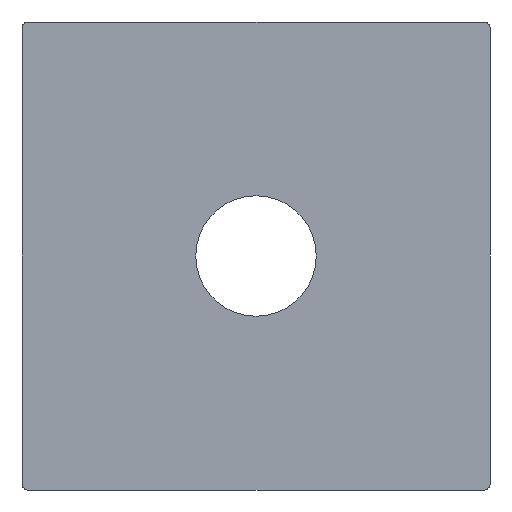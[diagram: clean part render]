
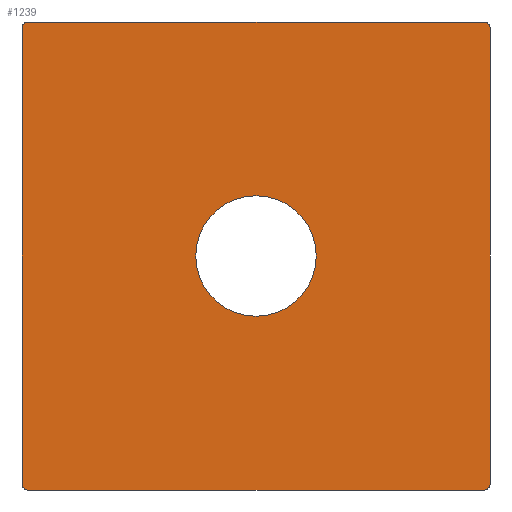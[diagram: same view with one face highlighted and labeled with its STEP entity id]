
A CAD part, front view. The second image highlights one B-rep face of the part: STEP entity #1239.
In plain terms, the highlighted planar face has unit normal (0, -1, 0).
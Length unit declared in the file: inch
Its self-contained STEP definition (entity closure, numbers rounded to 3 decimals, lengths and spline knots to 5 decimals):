
#50=PLANE('',#1346);
#110=LINE('',#2103,#209);
#111=LINE('',#2105,#210);
#148=LINE('',#2323,#247);
#149=LINE('',#2325,#248);
#209=VECTOR('',#1490,0.3937);
#210=VECTOR('',#1493,0.3937);
#247=VECTOR('',#1616,0.3937);
#248=VECTOR('',#1619,0.3937);
#318=FACE_BOUND('',#467,.T.);
#390=FACE_OUTER_BOUND('',#466,.T.);
#466=EDGE_LOOP('',(#1138,#1139,#1140,#1141,#1142,#1143,#1144,#1145));
#467=EDGE_LOOP('',(#1146));
#469=CIRCLE('',#1262,0.2575);
#473=CIRCLE('',#1277,0.025);
#477=CIRCLE('',#1283,0.025);
#481=CIRCLE('',#1289,0.025);
#485=CIRCLE('',#1296,0.025);
#499=VERTEX_POINT('',#1626);
#557=VERTEX_POINT('',#2046);
#558=VERTEX_POINT('',#2047);
#562=VERTEX_POINT('',#2059);
#563=VERTEX_POINT('',#2060);
#567=VERTEX_POINT('',#2072);
#568=VERTEX_POINT('',#2073);
#572=VERTEX_POINT('',#2088);
#573=VERTEX_POINT('',#2089);
#611=EDGE_CURVE('',#499,#499,#469,.T.);
#696=EDGE_CURVE('',#557,#558,#473,.T.);
#702=EDGE_CURVE('',#562,#563,#477,.T.);
#708=EDGE_CURVE('',#567,#568,#481,.T.);
#716=EDGE_CURVE('',#572,#573,#485,.T.);
#725=EDGE_CURVE('',#557,#568,#110,.T.);
#726=EDGE_CURVE('',#567,#573,#111,.T.);
#787=EDGE_CURVE('',#562,#558,#148,.T.);
#788=EDGE_CURVE('',#572,#563,#149,.T.);
#1138=ORIENTED_EDGE('',*,*,#696,.F.);
#1139=ORIENTED_EDGE('',*,*,#725,.T.);
#1140=ORIENTED_EDGE('',*,*,#708,.F.);
#1141=ORIENTED_EDGE('',*,*,#726,.T.);
#1142=ORIENTED_EDGE('',*,*,#716,.F.);
#1143=ORIENTED_EDGE('',*,*,#788,.T.);
#1144=ORIENTED_EDGE('',*,*,#702,.F.);
#1145=ORIENTED_EDGE('',*,*,#787,.T.);
#1146=ORIENTED_EDGE('',*,*,#611,.T.);
#1239=ADVANCED_FACE('',(#390,#318),#50,.F.);
#1262=AXIS2_PLACEMENT_3D('',#1627,#1353,#1354);
#1277=AXIS2_PLACEMENT_3D('',#2048,#1426,#1427);
#1283=AXIS2_PLACEMENT_3D('',#2061,#1440,#1441);
#1289=AXIS2_PLACEMENT_3D('',#2074,#1454,#1455);
#1296=AXIS2_PLACEMENT_3D('',#2090,#1472,#1473);
#1346=AXIS2_PLACEMENT_3D('',#2326,#1620,#1621);
#1353=DIRECTION('center_axis',(0.,1.,0.));
#1354=DIRECTION('ref_axis',(-1.,0.,0.));
#1426=DIRECTION('center_axis',(0.,1.,0.));
#1427=DIRECTION('ref_axis',(-0.707,0.,-0.707));
#1440=DIRECTION('center_axis',(0.,1.,0.));
#1441=DIRECTION('ref_axis',(-0.707,0.,0.707));
#1454=DIRECTION('center_axis',(0.,1.,0.));
#1455=DIRECTION('ref_axis',(0.707,0.,-0.707));
#1472=DIRECTION('center_axis',(0.,1.,0.));
#1473=DIRECTION('ref_axis',(0.707,0.,0.707));
#1490=DIRECTION('',(1.,0.,0.));
#1493=DIRECTION('',(0.,0.,1.));
#1616=DIRECTION('',(0.,0.,-1.));
#1619=DIRECTION('',(-1.,0.,0.));
#1620=DIRECTION('center_axis',(0.,1.,0.));
#1621=DIRECTION('ref_axis',(0.,0.,1.));
#1626=CARTESIAN_POINT('',(-0.7425,0.,-1.));
#1627=CARTESIAN_POINT('Origin',(-1.,0.,-1.));
#2046=CARTESIAN_POINT('',(-1.975,0.,-2.));
#2047=CARTESIAN_POINT('',(-2.,0.,-1.975));
#2048=CARTESIAN_POINT('Origin',(-1.975,0.,-1.975));
#2059=CARTESIAN_POINT('',(-2.,0.,-0.025));
#2060=CARTESIAN_POINT('',(-1.975,0.,0.));
#2061=CARTESIAN_POINT('Origin',(-1.975,0.,-0.025));
#2072=CARTESIAN_POINT('',(0.,0.,-1.975));
#2073=CARTESIAN_POINT('',(-0.025,0.,-2.));
#2074=CARTESIAN_POINT('Origin',(-0.025,0.,-1.975));
#2088=CARTESIAN_POINT('',(-0.025,0.,0.));
#2089=CARTESIAN_POINT('',(0.,0.,-0.025));
#2090=CARTESIAN_POINT('Origin',(-0.025,0.,-0.025));
#2103=CARTESIAN_POINT('',(-2.,0.,-2.));
#2105=CARTESIAN_POINT('',(0.,0.,-2.));
#2323=CARTESIAN_POINT('',(-2.,0.,0.));
#2325=CARTESIAN_POINT('',(0.,0.,0.));
#2326=CARTESIAN_POINT('Origin',(-1.,0.,-1.));
